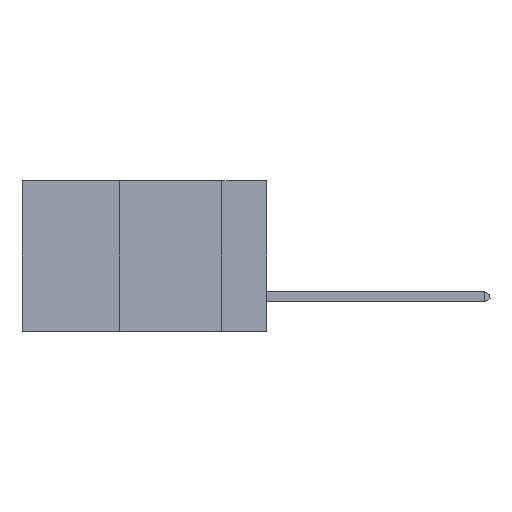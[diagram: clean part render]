
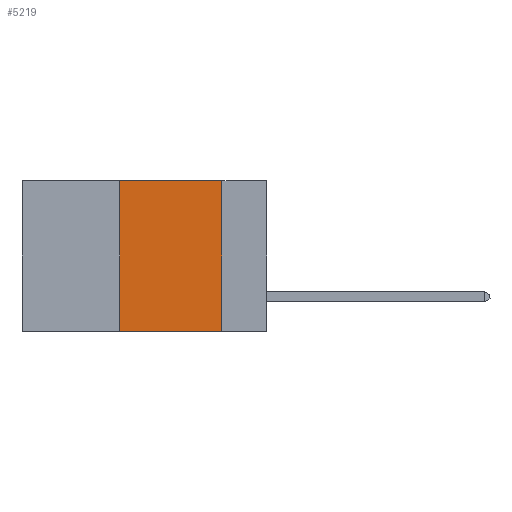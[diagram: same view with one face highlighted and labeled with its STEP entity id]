
A CAD part, left-side view. The second image highlights one B-rep face of the part: STEP entity #5219.
In plain terms, the highlighted planar face has unit normal (-1, 0, 0).
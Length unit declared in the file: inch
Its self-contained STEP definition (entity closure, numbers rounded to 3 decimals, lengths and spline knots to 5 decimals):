
#690 = VECTOR ( 'NONE', #3630, 39.37008 ) ;
#1335 = EDGE_CURVE ( 'NONE', #13975, #12610, #1683, .T. ) ;
#1605 = EDGE_CURVE ( 'NONE', #3006, #13975, #12736, .T. ) ;
#1683 = LINE ( 'NONE', #11441, #690 ) ;
#2129 = PLANE ( 'NONE',  #15189 ) ;
#3006 = VERTEX_POINT ( 'NONE', #10147 ) ;
#3321 = CARTESIAN_POINT ( 'NONE',  ( 0., 0.36, -0.37 ) ) ;
#3466 = LINE ( 'NONE', #13231, #14254 ) ;
#3630 = DIRECTION ( 'NONE',  ( 0., 0., -1. ) ) ;
#5179 = CARTESIAN_POINT ( 'NONE',  ( 0., 0.11, -0.37 ) ) ;
#5219 = ADVANCED_FACE ( 'NONE', ( #14912 ), #2129, .F. ) ;
#5390 = DIRECTION ( 'NONE',  ( 0., -1., 0. ) ) ;
#5858 = EDGE_CURVE ( 'NONE', #7327, #12610, #3466, .T. ) ;
#6446 = VECTOR ( 'NONE', #7778, 39.37008 ) ;
#7202 = DIRECTION ( 'NONE',  ( 0., -1., 0. ) ) ;
#7327 = VERTEX_POINT ( 'NONE', #3321 ) ;
#7465 = DIRECTION ( 'NONE',  ( 0., 0., -1. ) ) ;
#7492 = CARTESIAN_POINT ( 'NONE',  ( 0., 0.11, 0. ) ) ;
#7625 = ORIENTED_EDGE ( 'NONE', *, *, #1605, .F. ) ;
#7773 = ORIENTED_EDGE ( 'NONE', *, *, #1335, .F. ) ;
#7778 = DIRECTION ( 'NONE',  ( 0., 0., 1. ) ) ;
#8037 = ORIENTED_EDGE ( 'NONE', *, *, #5858, .T. ) ;
#9398 = VECTOR ( 'NONE', #7202, 39.37008 ) ;
#9928 = LINE ( 'NONE', #11585, #6446 ) ;
#10147 = CARTESIAN_POINT ( 'NONE',  ( 0., 0.36, 0. ) ) ;
#10950 = ORIENTED_EDGE ( 'NONE', *, *, #12546, .F. ) ;
#11093 = CARTESIAN_POINT ( 'NONE',  ( 0., 0.6, 0. ) ) ;
#11441 = CARTESIAN_POINT ( 'NONE',  ( 0., 0.11, 0. ) ) ;
#11585 = CARTESIAN_POINT ( 'NONE',  ( 0., 0.36, 0. ) ) ;
#12546 = EDGE_CURVE ( 'NONE', #7327, #3006, #9928, .T. ) ;
#12610 = VERTEX_POINT ( 'NONE', #5179 ) ;
#12736 = LINE ( 'NONE', #15057, #9398 ) ;
#13231 = CARTESIAN_POINT ( 'NONE',  ( 0., 0.6, -0.37 ) ) ;
#13975 = VERTEX_POINT ( 'NONE', #7492 ) ;
#14254 = VECTOR ( 'NONE', #5390, 39.37008 ) ;
#14912 = FACE_OUTER_BOUND ( 'NONE', #16437, .T. ) ;
#15057 = CARTESIAN_POINT ( 'NONE',  ( 0., 0.6, 0. ) ) ;
#15189 = AXIS2_PLACEMENT_3D ( 'NONE', #11093, #16418, #7465 ) ;
#16418 = DIRECTION ( 'NONE',  ( 1., 0., 0. ) ) ;
#16437 = EDGE_LOOP ( 'NONE', ( #7773, #7625, #10950, #8037 ) ) ;
